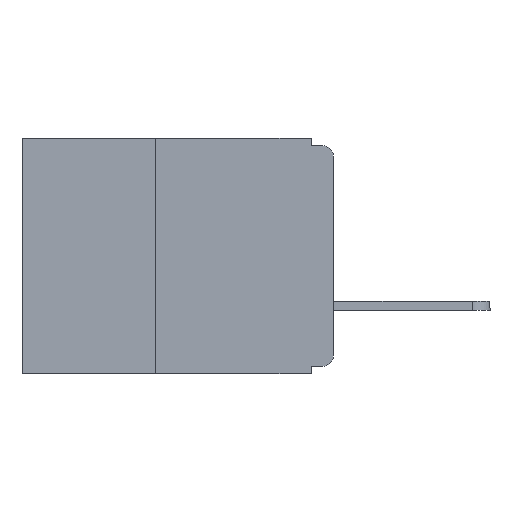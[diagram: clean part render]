
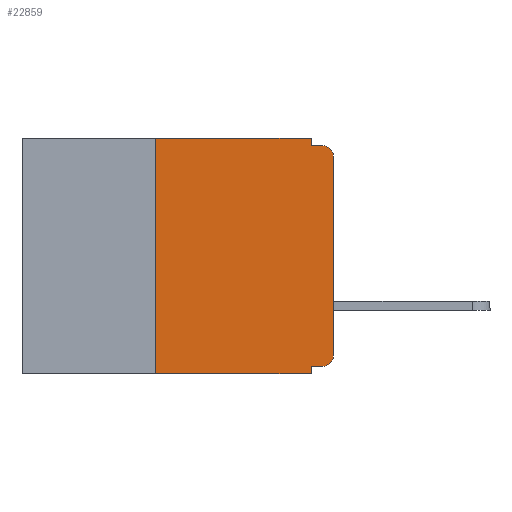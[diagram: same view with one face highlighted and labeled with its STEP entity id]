
A CAD part, left-side view. The second image highlights one B-rep face of the part: STEP entity #22859.
In plain terms, the highlighted planar face has unit normal (-1, 0, 0).
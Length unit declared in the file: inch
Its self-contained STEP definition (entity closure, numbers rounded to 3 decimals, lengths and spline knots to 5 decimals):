
#112 = ORIENTED_EDGE ( 'NONE', *, *, #16667, .F. ) ;
#349 = EDGE_CURVE ( 'NONE', #3388, #6494, #23428, .T. ) ;
#1654 = EDGE_CURVE ( 'NONE', #24027, #28264, #24112, .T. ) ;
#2188 = VECTOR ( 'NONE', #3223, 39.37008 ) ;
#2564 = CARTESIAN_POINT ( 'NONE',  ( 0., 0.031, 0. ) ) ;
#3223 = DIRECTION ( 'NONE',  ( 0., -1., 0. ) ) ;
#3276 = LINE ( 'NONE', #25934, #28815 ) ;
#3388 = VERTEX_POINT ( 'NONE', #6419 ) ;
#4068 = CARTESIAN_POINT ( 'NONE',  ( 0., 0.031, -0.32 ) ) ;
#4577 = ORIENTED_EDGE ( 'NONE', *, *, #20112, .T. ) ;
#4679 = CARTESIAN_POINT ( 'NONE',  ( 0., 0., -0.305 ) ) ;
#4834 = EDGE_CURVE ( 'NONE', #32859, #9708, #22787, .T. ) ;
#5759 = ORIENTED_EDGE ( 'NONE', *, *, #27154, .F. ) ;
#6285 = VECTOR ( 'NONE', #28352, 39.37008 ) ;
#6419 = CARTESIAN_POINT ( 'NONE',  ( 0., 0.25, -0.33 ) ) ;
#6494 = VERTEX_POINT ( 'NONE', #26015 ) ;
#7127 = LINE ( 'NONE', #13219, #6285 ) ;
#7283 = EDGE_CURVE ( 'NONE', #28264, #32859, #30526, .T. ) ;
#7345 = AXIS2_PLACEMENT_3D ( 'NONE', #25391, #25382, #25351 ) ;
#7682 = LINE ( 'NONE', #7977, #27225 ) ;
#7977 = CARTESIAN_POINT ( 'NONE',  ( 0., 0., -0.32 ) ) ;
#8606 = ORIENTED_EDGE ( 'NONE', *, *, #7283, .T. ) ;
#9113 = LINE ( 'NONE', #26074, #2188 ) ;
#9119 = PLANE ( 'NONE',  #30896 ) ;
#9708 = VERTEX_POINT ( 'NONE', #28466 ) ;
#10243 = EDGE_LOOP ( 'NONE', ( #8606, #10252, #23833, #5759, #12642, #22684, #4577, #11459, #112, #13885 ) ) ;
#10252 = ORIENTED_EDGE ( 'NONE', *, *, #4834, .T. ) ;
#11459 = ORIENTED_EDGE ( 'NONE', *, *, #13258, .F. ) ;
#11710 = DIRECTION ( 'NONE',  ( 0., 0., -1. ) ) ;
#11932 = FACE_OUTER_BOUND ( 'NONE', #10243, .T. ) ;
#12087 = CARTESIAN_POINT ( 'NONE',  ( 0., 0.015, -0.32 ) ) ;
#12642 = ORIENTED_EDGE ( 'NONE', *, *, #15740, .F. ) ;
#13073 = CARTESIAN_POINT ( 'NONE',  ( 0., 0.031, 0. ) ) ;
#13219 = CARTESIAN_POINT ( 'NONE',  ( 0., 0.031, -0.33 ) ) ;
#13258 = EDGE_CURVE ( 'NONE', #16591, #17898, #7127, .T. ) ;
#13885 = ORIENTED_EDGE ( 'NONE', *, *, #1654, .T. ) ;
#13957 = AXIS2_PLACEMENT_3D ( 'NONE', #16256, #16227, #30575 ) ;
#15740 = EDGE_CURVE ( 'NONE', #6494, #26584, #3276, .T. ) ;
#15872 = DIRECTION ( 'NONE',  ( 0., -1., 0. ) ) ;
#16227 = DIRECTION ( 'NONE',  ( -1., 0., 0. ) ) ;
#16256 = CARTESIAN_POINT ( 'NONE',  ( 0., 0.015, -0.305 ) ) ;
#16591 = VERTEX_POINT ( 'NONE', #4068 ) ;
#16658 = VECTOR ( 'NONE', #19942, 39.37008 ) ;
#16667 = EDGE_CURVE ( 'NONE', #24027, #16591, #7682, .T. ) ;
#16787 = CARTESIAN_POINT ( 'NONE',  ( 0., 0.437, 0. ) ) ;
#17898 = VERTEX_POINT ( 'NONE', #30703 ) ;
#18733 = CARTESIAN_POINT ( 'NONE',  ( 0., 0.25, -0.33 ) ) ;
#19942 = DIRECTION ( 'NONE',  ( 0., 0., 1. ) ) ;
#20112 = EDGE_CURVE ( 'NONE', #3388, #17898, #30626, .T. ) ;
#21285 = DIRECTION ( 'NONE',  ( 0., 0., 1. ) ) ;
#21494 = CARTESIAN_POINT ( 'NONE',  ( 0., 0., 0. ) ) ;
#22676 = EDGE_CURVE ( 'NONE', #31628, #9708, #9113, .T. ) ;
#22684 = ORIENTED_EDGE ( 'NONE', *, *, #349, .F. ) ;
#22787 = CIRCLE ( 'NONE', #7345, 0.015 ) ;
#22859 = ADVANCED_FACE ( 'NONE', ( #11932 ), #9119, .F. ) ;
#23280 = VECTOR ( 'NONE', #24113, 39.37008 ) ;
#23428 = LINE ( 'NONE', #18733, #16658 ) ;
#23833 = ORIENTED_EDGE ( 'NONE', *, *, #22676, .F. ) ;
#23948 = VECTOR ( 'NONE', #21285, 39.37008 ) ;
#24027 = VERTEX_POINT ( 'NONE', #12087 ) ;
#24112 = CIRCLE ( 'NONE', #13957, 0.015 ) ;
#24113 = DIRECTION ( 'NONE',  ( 0., -1., 0. ) ) ;
#24489 = VECTOR ( 'NONE', #28222, 39.37008 ) ;
#25351 = DIRECTION ( 'NONE',  ( 0., 0., -1. ) ) ;
#25382 = DIRECTION ( 'NONE',  ( -1., 0., 0. ) ) ;
#25391 = CARTESIAN_POINT ( 'NONE',  ( 0., 0.015, -0.025 ) ) ;
#25556 = CARTESIAN_POINT ( 'NONE',  ( 0., 0.031, -0.01 ) ) ;
#25934 = CARTESIAN_POINT ( 'NONE',  ( 0., 0.437, 0. ) ) ;
#26015 = CARTESIAN_POINT ( 'NONE',  ( 0., 0.25, 0. ) ) ;
#26074 = CARTESIAN_POINT ( 'NONE',  ( 0., 0., -0.01 ) ) ;
#26584 = VERTEX_POINT ( 'NONE', #2564 ) ;
#26601 = CARTESIAN_POINT ( 'NONE',  ( 0., 0.437, -0.33 ) ) ;
#26919 = DIRECTION ( 'NONE',  ( 1., 0., 0. ) ) ;
#27154 = EDGE_CURVE ( 'NONE', #26584, #31628, #30267, .T. ) ;
#27225 = VECTOR ( 'NONE', #28307, 39.37008 ) ;
#28222 = DIRECTION ( 'NONE',  ( 0., 0., -1. ) ) ;
#28264 = VERTEX_POINT ( 'NONE', #4679 ) ;
#28290 = CARTESIAN_POINT ( 'NONE',  ( 0., 0., -0.025 ) ) ;
#28307 = DIRECTION ( 'NONE',  ( 0., 1., 0. ) ) ;
#28352 = DIRECTION ( 'NONE',  ( 0., 0., -1. ) ) ;
#28466 = CARTESIAN_POINT ( 'NONE',  ( 0., 0.015, -0.01 ) ) ;
#28815 = VECTOR ( 'NONE', #15872, 39.37008 ) ;
#30267 = LINE ( 'NONE', #13073, #24489 ) ;
#30526 = LINE ( 'NONE', #21494, #23948 ) ;
#30575 = DIRECTION ( 'NONE',  ( 0., 0., -1. ) ) ;
#30626 = LINE ( 'NONE', #26601, #23280 ) ;
#30703 = CARTESIAN_POINT ( 'NONE',  ( 0., 0.031, -0.33 ) ) ;
#30896 = AXIS2_PLACEMENT_3D ( 'NONE', #16787, #26919, #11710 ) ;
#31628 = VERTEX_POINT ( 'NONE', #25556 ) ;
#32859 = VERTEX_POINT ( 'NONE', #28290 ) ;
